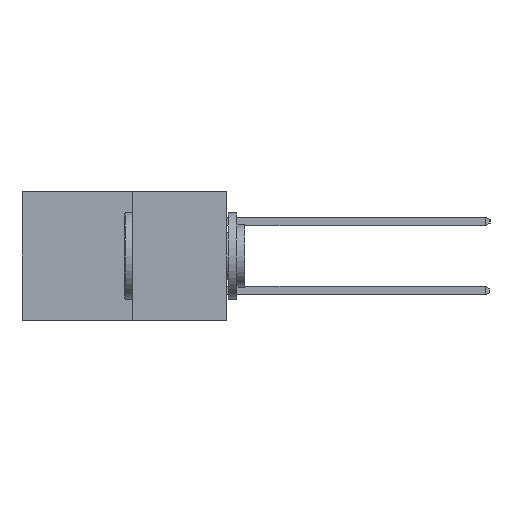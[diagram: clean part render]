
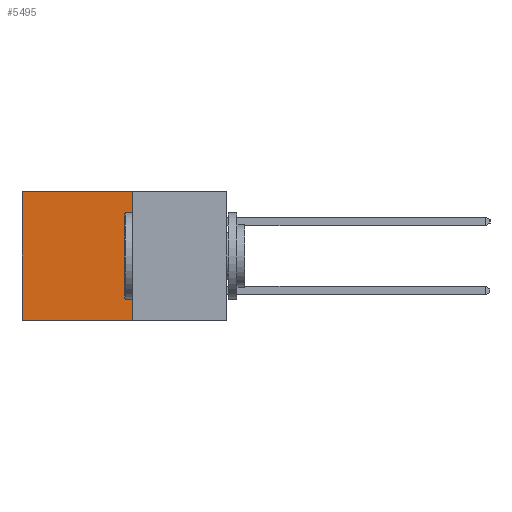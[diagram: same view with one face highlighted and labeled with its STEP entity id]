
A CAD part, left-side view. The second image highlights one B-rep face of the part: STEP entity #5495.
In plain terms, the highlighted planar face has unit normal (-1, 0, 0).
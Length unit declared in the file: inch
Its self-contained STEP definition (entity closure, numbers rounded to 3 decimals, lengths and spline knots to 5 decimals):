
#266 = EDGE_CURVE ( 'NONE', #2731, #881, #4908, .T. ) ;
#669 = DIRECTION ( 'NONE',  ( 0., 1., 0. ) ) ;
#881 = VERTEX_POINT ( 'NONE', #2355 ) ;
#1207 = EDGE_CURVE ( 'NONE', #2578, #2811, #3957, .T. ) ;
#1221 = EDGE_CURVE ( 'NONE', #881, #2811, #1848, .T. ) ;
#1244 = CARTESIAN_POINT ( 'NONE',  ( 0.277, 0.27, -0.37 ) ) ;
#1325 = EDGE_LOOP ( 'NONE', ( #3952, #5740, #8207, #4591 ) ) ;
#1578 = EDGE_CURVE ( 'NONE', #2731, #2578, #7336, .T. ) ;
#1732 = CARTESIAN_POINT ( 'NONE',  ( 0.277, 0.59, -0.37 ) ) ;
#1848 = LINE ( 'NONE', #7619, #5345 ) ;
#1883 = CARTESIAN_POINT ( 'NONE',  ( 0.277, 0.59, 0. ) ) ;
#2355 = CARTESIAN_POINT ( 'NONE',  ( 0.277, 0.27, -0.37 ) ) ;
#2578 = VERTEX_POINT ( 'NONE', #1883 ) ;
#2731 = VERTEX_POINT ( 'NONE', #3583 ) ;
#2811 = VERTEX_POINT ( 'NONE', #1732 ) ;
#3190 = FACE_OUTER_BOUND ( 'NONE', #1325, .T. ) ;
#3583 = CARTESIAN_POINT ( 'NONE',  ( 0.277, 0.27, 0. ) ) ;
#3737 = VECTOR ( 'NONE', #7187, 39.37008 ) ;
#3952 = ORIENTED_EDGE ( 'NONE', *, *, #1207, .T. ) ;
#3957 = LINE ( 'NONE', #4271, #3737 ) ;
#4033 = DIRECTION ( 'NONE',  ( 0., 0., -1. ) ) ;
#4035 = DIRECTION ( 'NONE',  ( 1., 0., 0. ) ) ;
#4065 = CARTESIAN_POINT ( 'NONE',  ( 0.277, 0.27, -0.37 ) ) ;
#4117 = PLANE ( 'NONE',  #5303 ) ;
#4271 = CARTESIAN_POINT ( 'NONE',  ( 0.277, 0.59, -0.37 ) ) ;
#4430 = DIRECTION ( 'NONE',  ( 0., 0., -1. ) ) ;
#4591 = ORIENTED_EDGE ( 'NONE', *, *, #1578, .T. ) ;
#4908 = LINE ( 'NONE', #1244, #8100 ) ;
#5172 = CARTESIAN_POINT ( 'NONE',  ( 0.277, 0.27, 0. ) ) ;
#5303 = AXIS2_PLACEMENT_3D ( 'NONE', #4065, #4035, #4033 ) ;
#5345 = VECTOR ( 'NONE', #7569, 39.37008 ) ;
#5437 = VECTOR ( 'NONE', #669, 39.37008 ) ;
#5495 = ADVANCED_FACE ( 'NONE', ( #3190 ), #4117, .F. ) ;
#5740 = ORIENTED_EDGE ( 'NONE', *, *, #1221, .F. ) ;
#7187 = DIRECTION ( 'NONE',  ( 0., 0., -1. ) ) ;
#7336 = LINE ( 'NONE', #5172, #5437 ) ;
#7569 = DIRECTION ( 'NONE',  ( 0., 1., 0. ) ) ;
#7619 = CARTESIAN_POINT ( 'NONE',  ( 0.277, 0.27, -0.37 ) ) ;
#8100 = VECTOR ( 'NONE', #4430, 39.37008 ) ;
#8207 = ORIENTED_EDGE ( 'NONE', *, *, #266, .F. ) ;
